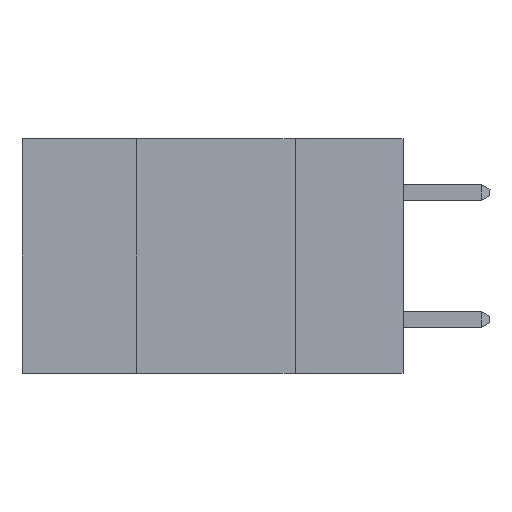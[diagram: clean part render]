
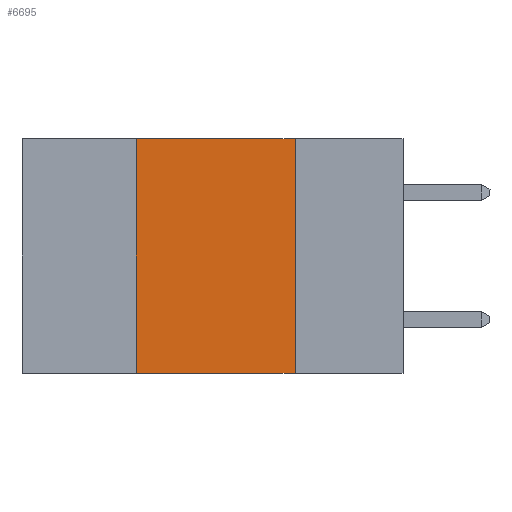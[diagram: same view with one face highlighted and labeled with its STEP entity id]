
A CAD part, left-side view. The second image highlights one B-rep face of the part: STEP entity #6695.
In plain terms, the highlighted planar face has unit normal (-1, 0, 0).
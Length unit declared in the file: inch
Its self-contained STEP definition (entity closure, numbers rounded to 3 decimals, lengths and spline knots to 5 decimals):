
#219 = VERTEX_POINT ( 'NONE', #5869 ) ;
#853 = DIRECTION ( 'NONE',  ( 0., -1., 0. ) ) ;
#886 = CARTESIAN_POINT ( 'NONE',  ( 0., 0.6, -0.37 ) ) ;
#963 = CARTESIAN_POINT ( 'NONE',  ( 0., 0.6, 0. ) ) ;
#1139 = CARTESIAN_POINT ( 'NONE',  ( 0., 0.42, 0. ) ) ;
#1789 = EDGE_CURVE ( 'NONE', #6426, #4709, #10786, .T. ) ;
#1929 = CARTESIAN_POINT ( 'NONE',  ( 0., 0.17, 0. ) ) ;
#2080 = EDGE_LOOP ( 'NONE', ( #2215, #8914, #9161, #2749 ) ) ;
#2215 = ORIENTED_EDGE ( 'NONE', *, *, #5276, .F. ) ;
#2251 = LINE ( 'NONE', #10877, #6489 ) ;
#2689 = LINE ( 'NONE', #1139, #3217 ) ;
#2743 = PLANE ( 'NONE',  #6917 ) ;
#2749 = ORIENTED_EDGE ( 'NONE', *, *, #1789, .T. ) ;
#3217 = VECTOR ( 'NONE', #7255, 39.37008 ) ;
#3775 = CARTESIAN_POINT ( 'NONE',  ( 0., 0.17, -0.37 ) ) ;
#4098 = EDGE_CURVE ( 'NONE', #6426, #219, #2689, .T. ) ;
#4709 = VERTEX_POINT ( 'NONE', #3775 ) ;
#5276 = EDGE_CURVE ( 'NONE', #6239, #4709, #8956, .T. ) ;
#5343 = DIRECTION ( 'NONE',  ( 0., 0., -1. ) ) ;
#5359 = DIRECTION ( 'NONE',  ( 0., 0., -1. ) ) ;
#5766 = EDGE_CURVE ( 'NONE', #219, #6239, #2251, .T. ) ;
#5841 = FACE_OUTER_BOUND ( 'NONE', #2080, .T. ) ;
#5869 = CARTESIAN_POINT ( 'NONE',  ( 0., 0.42, 0. ) ) ;
#6239 = VERTEX_POINT ( 'NONE', #9888 ) ;
#6426 = VERTEX_POINT ( 'NONE', #10092 ) ;
#6478 = VECTOR ( 'NONE', #7759, 39.37008 ) ;
#6489 = VECTOR ( 'NONE', #853, 39.37008 ) ;
#6695 = ADVANCED_FACE ( 'NONE', ( #5841 ), #2743, .F. ) ;
#6917 = AXIS2_PLACEMENT_3D ( 'NONE', #963, #10197, #5343 ) ;
#7023 = VECTOR ( 'NONE', #5359, 39.37008 ) ;
#7255 = DIRECTION ( 'NONE',  ( 0., 0., 1. ) ) ;
#7759 = DIRECTION ( 'NONE',  ( 0., -1., 0. ) ) ;
#8914 = ORIENTED_EDGE ( 'NONE', *, *, #5766, .F. ) ;
#8956 = LINE ( 'NONE', #1929, #7023 ) ;
#9161 = ORIENTED_EDGE ( 'NONE', *, *, #4098, .F. ) ;
#9888 = CARTESIAN_POINT ( 'NONE',  ( 0., 0.17, 0. ) ) ;
#10092 = CARTESIAN_POINT ( 'NONE',  ( 0., 0.42, -0.37 ) ) ;
#10197 = DIRECTION ( 'NONE',  ( 1., 0., 0. ) ) ;
#10786 = LINE ( 'NONE', #886, #6478 ) ;
#10877 = CARTESIAN_POINT ( 'NONE',  ( 0., 0.6, 0. ) ) ;
